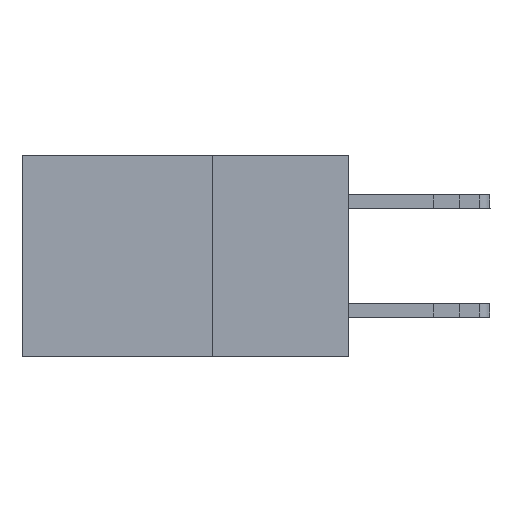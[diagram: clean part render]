
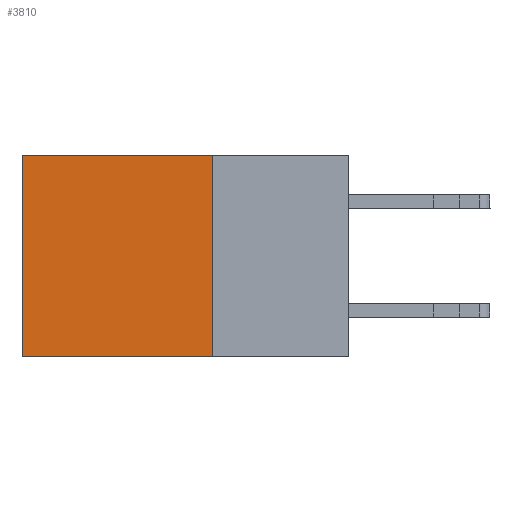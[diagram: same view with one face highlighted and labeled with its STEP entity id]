
A CAD part, left-side view. The second image highlights one B-rep face of the part: STEP entity #3810.
In plain terms, the highlighted planar face has unit normal (-1, 0, 0).
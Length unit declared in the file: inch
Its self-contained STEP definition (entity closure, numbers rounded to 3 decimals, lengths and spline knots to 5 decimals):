
#310 = LINE ( 'NONE', #11938, #12618 ) ;
#343 = ORIENTED_EDGE ( 'NONE', *, *, #14789, .T. ) ;
#1695 = DIRECTION ( 'NONE',  ( 0., 0., -1. ) ) ;
#2306 = PLANE ( 'NONE',  #2896 ) ;
#2410 = FACE_OUTER_BOUND ( 'NONE', #9549, .T. ) ;
#2896 = AXIS2_PLACEMENT_3D ( 'NONE', #8268, #6795, #6887 ) ;
#3152 = CARTESIAN_POINT ( 'NONE',  ( 0.2615, 0.6, -0.37 ) ) ;
#3354 = ORIENTED_EDGE ( 'NONE', *, *, #12906, .T. ) ;
#3612 = VERTEX_POINT ( 'NONE', #10506 ) ;
#3810 = ADVANCED_FACE ( 'NONE', ( #2410 ), #2306, .F. ) ;
#5295 = VERTEX_POINT ( 'NONE', #11774 ) ;
#5891 = EDGE_CURVE ( 'NONE', #5295, #15902, #310, .T. ) ;
#6261 = DIRECTION ( 'NONE',  ( 0., 1., 0. ) ) ;
#6293 = VECTOR ( 'NONE', #6582, 39.37008 ) ;
#6582 = DIRECTION ( 'NONE',  ( 0., 0., -1. ) ) ;
#6795 = DIRECTION ( 'NONE',  ( 1., 0., 0. ) ) ;
#6887 = DIRECTION ( 'NONE',  ( 0., 0., -1. ) ) ;
#8062 = LINE ( 'NONE', #13999, #6293 ) ;
#8268 = CARTESIAN_POINT ( 'NONE',  ( 0.2615, 0.25, -0.37 ) ) ;
#8446 = ORIENTED_EDGE ( 'NONE', *, *, #5891, .F. ) ;
#9549 = EDGE_LOOP ( 'NONE', ( #343, #8446, #18347, #3354 ) ) ;
#10102 = CARTESIAN_POINT ( 'NONE',  ( 0.2615, 0.25, 0. ) ) ;
#10358 = VERTEX_POINT ( 'NONE', #13729 ) ;
#10506 = CARTESIAN_POINT ( 'NONE',  ( 0.2615, 0.6, 0. ) ) ;
#11774 = CARTESIAN_POINT ( 'NONE',  ( 0.2615, 0.25, -0.37 ) ) ;
#11938 = CARTESIAN_POINT ( 'NONE',  ( 0.2615, 0.25, -0.37 ) ) ;
#12034 = LINE ( 'NONE', #3152, #19084 ) ;
#12618 = VECTOR ( 'NONE', #6261, 39.37008 ) ;
#12906 = EDGE_CURVE ( 'NONE', #10358, #3612, #17623, .T. ) ;
#13729 = CARTESIAN_POINT ( 'NONE',  ( 0.2615, 0.25, 0. ) ) ;
#13999 = CARTESIAN_POINT ( 'NONE',  ( 0.2615, 0.25, -0.37 ) ) ;
#14549 = EDGE_CURVE ( 'NONE', #10358, #5295, #8062, .T. ) ;
#14789 = EDGE_CURVE ( 'NONE', #3612, #15902, #12034, .T. ) ;
#15902 = VERTEX_POINT ( 'NONE', #18844 ) ;
#17427 = DIRECTION ( 'NONE',  ( 0., 1., 0. ) ) ;
#17473 = VECTOR ( 'NONE', #17427, 39.37008 ) ;
#17623 = LINE ( 'NONE', #10102, #17473 ) ;
#18347 = ORIENTED_EDGE ( 'NONE', *, *, #14549, .F. ) ;
#18844 = CARTESIAN_POINT ( 'NONE',  ( 0.2615, 0.6, -0.37 ) ) ;
#19084 = VECTOR ( 'NONE', #1695, 39.37008 ) ;
